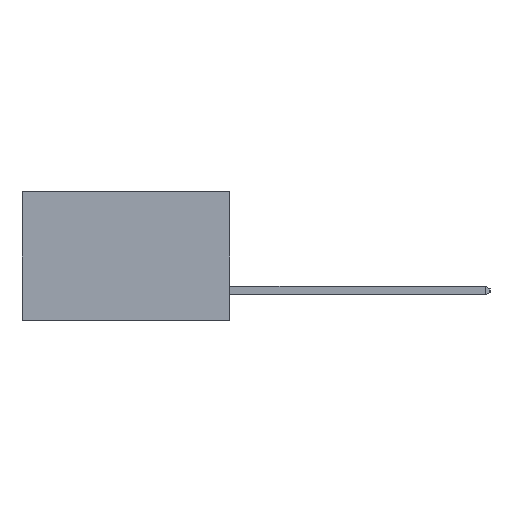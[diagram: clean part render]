
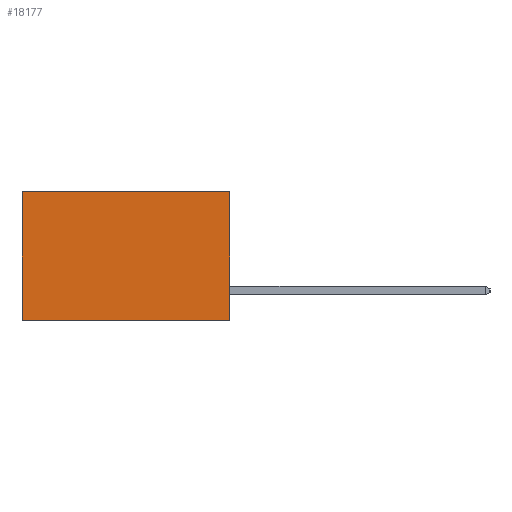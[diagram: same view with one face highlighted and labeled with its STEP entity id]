
A CAD part, left-side view. The second image highlights one B-rep face of the part: STEP entity #18177.
In plain terms, the highlighted planar face has unit normal (-1, 0, 0).
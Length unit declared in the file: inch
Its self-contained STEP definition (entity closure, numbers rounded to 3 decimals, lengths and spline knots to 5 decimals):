
#268 = ORIENTED_EDGE ( 'NONE', *, *, #3678, .F. ) ;
#296 = CARTESIAN_POINT ( 'NONE',  ( 0.2615, 0., -0.37 ) ) ;
#868 = DIRECTION ( 'NONE',  ( 1., 0., 0. ) ) ;
#1309 = EDGE_LOOP ( 'NONE', ( #13071, #268, #5984, #17982 ) ) ;
#1825 = VECTOR ( 'NONE', #15247, 39.37008 ) ;
#1851 = LINE ( 'NONE', #4218, #9409 ) ;
#2711 = CARTESIAN_POINT ( 'NONE',  ( 0.2615, 0., 0. ) ) ;
#2788 = VERTEX_POINT ( 'NONE', #18759 ) ;
#3006 = VECTOR ( 'NONE', #8731, 39.37008 ) ;
#3678 = EDGE_CURVE ( 'NONE', #8997, #5100, #13553, .T. ) ;
#4218 = CARTESIAN_POINT ( 'NONE',  ( 0.2615, 0., 0. ) ) ;
#4245 = AXIS2_PLACEMENT_3D ( 'NONE', #9945, #868, #11471 ) ;
#4318 = DIRECTION ( 'NONE',  ( 0., 1., 0. ) ) ;
#5100 = VERTEX_POINT ( 'NONE', #12840 ) ;
#5480 = EDGE_CURVE ( 'NONE', #15222, #2788, #1851, .T. ) ;
#5745 = CARTESIAN_POINT ( 'NONE',  ( 0.2615, 0., -0.37 ) ) ;
#5984 = ORIENTED_EDGE ( 'NONE', *, *, #18273, .F. ) ;
#7081 = LINE ( 'NONE', #5745, #3006 ) ;
#8731 = DIRECTION ( 'NONE',  ( 0., 0., -1. ) ) ;
#8922 = FACE_OUTER_BOUND ( 'NONE', #1309, .T. ) ;
#8997 = VERTEX_POINT ( 'NONE', #296 ) ;
#9331 = CARTESIAN_POINT ( 'NONE',  ( 0.2615, 0., -0.37 ) ) ;
#9409 = VECTOR ( 'NONE', #4318, 39.37008 ) ;
#9457 = EDGE_CURVE ( 'NONE', #2788, #5100, #17967, .T. ) ;
#9660 = DIRECTION ( 'NONE',  ( 0., 1., 0. ) ) ;
#9945 = CARTESIAN_POINT ( 'NONE',  ( 0.2615, 0., -0.37 ) ) ;
#11405 = PLANE ( 'NONE',  #4245 ) ;
#11471 = DIRECTION ( 'NONE',  ( 0., 0., -1. ) ) ;
#12840 = CARTESIAN_POINT ( 'NONE',  ( 0.2615, 0.6, -0.37 ) ) ;
#13071 = ORIENTED_EDGE ( 'NONE', *, *, #9457, .T. ) ;
#13072 = VECTOR ( 'NONE', #9660, 39.37008 ) ;
#13553 = LINE ( 'NONE', #9331, #13072 ) ;
#15222 = VERTEX_POINT ( 'NONE', #2711 ) ;
#15247 = DIRECTION ( 'NONE',  ( 0., 0., -1. ) ) ;
#15293 = CARTESIAN_POINT ( 'NONE',  ( 0.2615, 0.6, -0.37 ) ) ;
#17967 = LINE ( 'NONE', #15293, #1825 ) ;
#17982 = ORIENTED_EDGE ( 'NONE', *, *, #5480, .T. ) ;
#18177 = ADVANCED_FACE ( 'NONE', ( #8922 ), #11405, .F. ) ;
#18273 = EDGE_CURVE ( 'NONE', #15222, #8997, #7081, .T. ) ;
#18759 = CARTESIAN_POINT ( 'NONE',  ( 0.2615, 0.6, 0. ) ) ;
